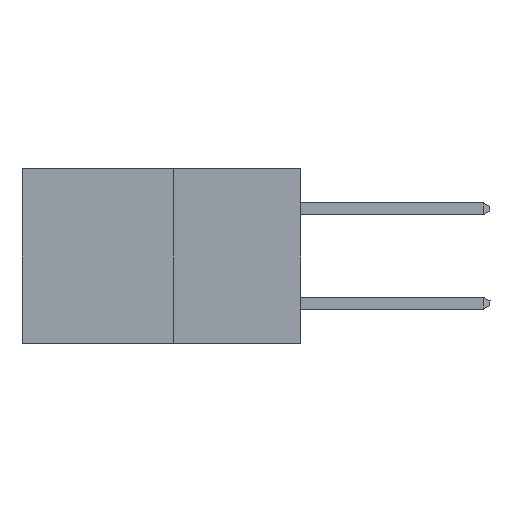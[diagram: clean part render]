
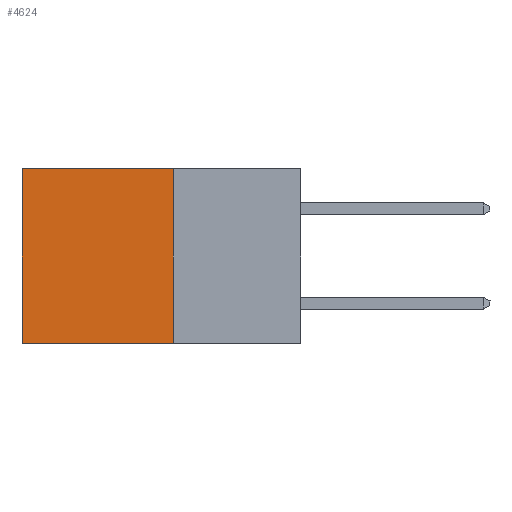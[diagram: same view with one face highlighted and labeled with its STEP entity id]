
A CAD part, left-side view. The second image highlights one B-rep face of the part: STEP entity #4624.
In plain terms, the highlighted planar face has unit normal (-1, 0, 0).
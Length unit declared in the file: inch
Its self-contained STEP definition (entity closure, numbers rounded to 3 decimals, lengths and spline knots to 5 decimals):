
#1395 = EDGE_CURVE ( 'NONE', #4477, #2114, #8247, .T. ) ;
#1487 = DIRECTION ( 'NONE',  ( 0., 0., -1. ) ) ;
#2114 = VERTEX_POINT ( 'NONE', #6823 ) ;
#2362 = AXIS2_PLACEMENT_3D ( 'NONE', #2533, #4769, #1487 ) ;
#2451 = FACE_OUTER_BOUND ( 'NONE', #10272, .T. ) ;
#2533 = CARTESIAN_POINT ( 'NONE',  ( 0.277, 0.27, -0.37 ) ) ;
#3270 = CARTESIAN_POINT ( 'NONE',  ( 0.277, 0.27, 0. ) ) ;
#3275 = DIRECTION ( 'NONE',  ( 0., 1., 0. ) ) ;
#3522 = LINE ( 'NONE', #3270, #5462 ) ;
#3815 = VECTOR ( 'NONE', #6831, 39.37008 ) ;
#4056 = LINE ( 'NONE', #8169, #5971 ) ;
#4240 = EDGE_CURVE ( 'NONE', #4477, #9759, #3522, .T. ) ;
#4470 = EDGE_CURVE ( 'NONE', #9759, #8813, #4056, .T. ) ;
#4476 = PLANE ( 'NONE',  #2362 ) ;
#4477 = VERTEX_POINT ( 'NONE', #7235 ) ;
#4528 = ORIENTED_EDGE ( 'NONE', *, *, #4470, .T. ) ;
#4624 = ADVANCED_FACE ( 'NONE', ( #2451 ), #4476, .F. ) ;
#4769 = DIRECTION ( 'NONE',  ( 1., 0., 0. ) ) ;
#5204 = ORIENTED_EDGE ( 'NONE', *, *, #9657, .F. ) ;
#5462 = VECTOR ( 'NONE', #3275, 39.37008 ) ;
#5938 = ORIENTED_EDGE ( 'NONE', *, *, #1395, .F. ) ;
#5971 = VECTOR ( 'NONE', #7605, 39.37008 ) ;
#6148 = ORIENTED_EDGE ( 'NONE', *, *, #4240, .T. ) ;
#6823 = CARTESIAN_POINT ( 'NONE',  ( 0.277, 0.27, -0.37 ) ) ;
#6831 = DIRECTION ( 'NONE',  ( 0., 0., -1. ) ) ;
#6849 = LINE ( 'NONE', #8951, #10277 ) ;
#7235 = CARTESIAN_POINT ( 'NONE',  ( 0.277, 0.27, 0. ) ) ;
#7499 = DIRECTION ( 'NONE',  ( 0., 1., 0. ) ) ;
#7605 = DIRECTION ( 'NONE',  ( 0., 0., -1. ) ) ;
#7714 = CARTESIAN_POINT ( 'NONE',  ( 0.277, 0.59, -0.37 ) ) ;
#8169 = CARTESIAN_POINT ( 'NONE',  ( 0.277, 0.59, -0.37 ) ) ;
#8247 = LINE ( 'NONE', #10043, #3815 ) ;
#8293 = CARTESIAN_POINT ( 'NONE',  ( 0.277, 0.59, 0. ) ) ;
#8813 = VERTEX_POINT ( 'NONE', #7714 ) ;
#8951 = CARTESIAN_POINT ( 'NONE',  ( 0.277, 0.27, -0.37 ) ) ;
#9657 = EDGE_CURVE ( 'NONE', #2114, #8813, #6849, .T. ) ;
#9759 = VERTEX_POINT ( 'NONE', #8293 ) ;
#10043 = CARTESIAN_POINT ( 'NONE',  ( 0.277, 0.27, -0.37 ) ) ;
#10272 = EDGE_LOOP ( 'NONE', ( #4528, #5204, #5938, #6148 ) ) ;
#10277 = VECTOR ( 'NONE', #7499, 39.37008 ) ;
